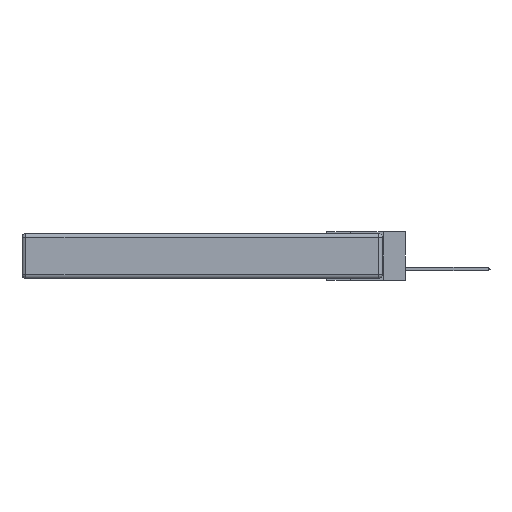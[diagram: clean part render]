
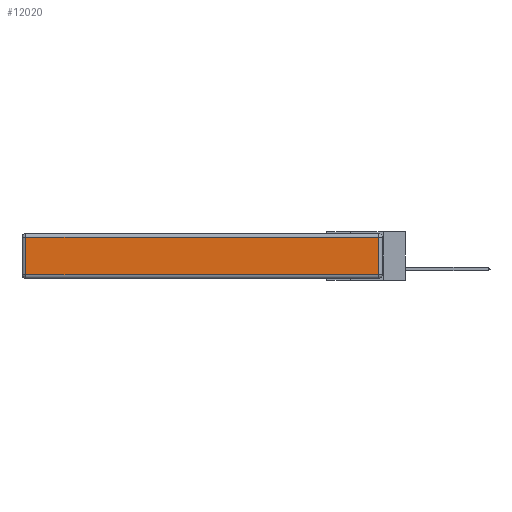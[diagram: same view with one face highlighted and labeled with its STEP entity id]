
A CAD part, left-side view. The second image highlights one B-rep face of the part: STEP entity #12020.
In plain terms, the highlighted planar face has unit normal (-1, 0, 0).
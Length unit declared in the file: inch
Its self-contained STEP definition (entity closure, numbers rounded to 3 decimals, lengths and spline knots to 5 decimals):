
#164 = CARTESIAN_POINT ( 'NONE',  ( 0., 0., -0.313 ) ) ;
#1476 = PLANE ( 'NONE',  #8801 ) ;
#1701 = VECTOR ( 'NONE', #4849, 39.37008 ) ;
#2914 = VERTEX_POINT ( 'NONE', #4818 ) ;
#3520 = LINE ( 'NONE', #13727, #9365 ) ;
#3541 = LINE ( 'NONE', #8645, #9005 ) ;
#4070 = EDGE_LOOP ( 'NONE', ( #9027, #14437, #13016, #7247 ) ) ;
#4716 = LINE ( 'NONE', #164, #8652 ) ;
#4818 = CARTESIAN_POINT ( 'NONE',  ( 0., 2.72, -0.03 ) ) ;
#4849 = DIRECTION ( 'NONE',  ( 0., 1., 0. ) ) ;
#5131 = DIRECTION ( 'NONE',  ( 0., 0., 1. ) ) ;
#5134 = VERTEX_POINT ( 'NONE', #11529 ) ;
#6175 = EDGE_CURVE ( 'NONE', #9011, #11161, #4716, .T. ) ;
#6864 = CARTESIAN_POINT ( 'NONE',  ( 0., 2.72, -0.313 ) ) ;
#7150 = EDGE_CURVE ( 'NONE', #11161, #5134, #3541, .T. ) ;
#7247 = ORIENTED_EDGE ( 'NONE', *, *, #7435, .T. ) ;
#7264 = CARTESIAN_POINT ( 'NONE',  ( 0., 2.75, -0.03 ) ) ;
#7435 = EDGE_CURVE ( 'NONE', #2914, #9011, #3520, .T. ) ;
#8645 = CARTESIAN_POINT ( 'NONE',  ( 0., 0.03, -0.343 ) ) ;
#8652 = VECTOR ( 'NONE', #13587, 39.37008 ) ;
#8801 = AXIS2_PLACEMENT_3D ( 'NONE', #11043, #11142, #5131 ) ;
#9005 = VECTOR ( 'NONE', #11118, 39.37008 ) ;
#9011 = VERTEX_POINT ( 'NONE', #6864 ) ;
#9027 = ORIENTED_EDGE ( 'NONE', *, *, #6175, .T. ) ;
#9365 = VECTOR ( 'NONE', #11360, 39.37008 ) ;
#11043 = CARTESIAN_POINT ( 'NONE',  ( 0., 0., -0.343 ) ) ;
#11076 = CARTESIAN_POINT ( 'NONE',  ( 0., 0.03, -0.313 ) ) ;
#11118 = DIRECTION ( 'NONE',  ( 0., 0., 1. ) ) ;
#11142 = DIRECTION ( 'NONE',  ( -1., 0., 0. ) ) ;
#11161 = VERTEX_POINT ( 'NONE', #11076 ) ;
#11360 = DIRECTION ( 'NONE',  ( 0., 0., -1. ) ) ;
#11529 = CARTESIAN_POINT ( 'NONE',  ( 0., 0.03, -0.03 ) ) ;
#11718 = LINE ( 'NONE', #7264, #1701 ) ;
#11919 = EDGE_CURVE ( 'NONE', #5134, #2914, #11718, .T. ) ;
#12020 = ADVANCED_FACE ( 'NONE', ( #12684 ), #1476, .T. ) ;
#12684 = FACE_OUTER_BOUND ( 'NONE', #4070, .T. ) ;
#13016 = ORIENTED_EDGE ( 'NONE', *, *, #11919, .T. ) ;
#13587 = DIRECTION ( 'NONE',  ( 0., -1., 0. ) ) ;
#13727 = CARTESIAN_POINT ( 'NONE',  ( 0., 2.72, -0.343 ) ) ;
#14437 = ORIENTED_EDGE ( 'NONE', *, *, #7150, .T. ) ;
